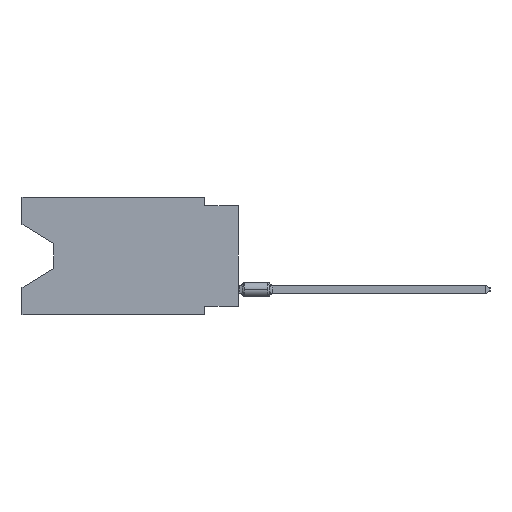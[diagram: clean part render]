
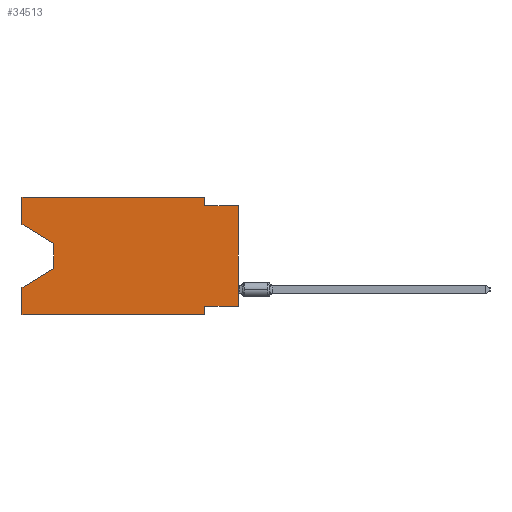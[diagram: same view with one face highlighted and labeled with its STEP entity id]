
A CAD part, left-side view. The second image highlights one B-rep face of the part: STEP entity #34513.
In plain terms, the highlighted planar face has unit normal (-1, 0, 0).
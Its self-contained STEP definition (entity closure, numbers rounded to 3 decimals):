
#129 = VECTOR ( 'NONE', #29697, 1000. ) ;
#216 = LINE ( 'NONE', #17724, #31245 ) ;
#1374 = VECTOR ( 'NONE', #54498, 1000. ) ;
#4129 = CARTESIAN_POINT ( 'NONE',  ( 0., 0., -8.255 ) ) ;
#4713 = CARTESIAN_POINT ( 'NONE',  ( 0., 16.383, -2.038 ) ) ;
#5659 = VERTEX_POINT ( 'NONE', #6612 ) ;
#6076 = EDGE_CURVE ( 'NONE', #41619, #32062, #18336, .T. ) ;
#6612 = CARTESIAN_POINT ( 'NONE',  ( 0., 13.97, -5.385 ) ) ;
#6839 = VERTEX_POINT ( 'NONE', #66470 ) ;
#8188 = LINE ( 'NONE', #26100, #9422 ) ;
#8651 = CARTESIAN_POINT ( 'NONE',  ( 0., 0., -0.635 ) ) ;
#9422 = VECTOR ( 'NONE', #55083, 1000. ) ;
#10755 = DIRECTION ( 'NONE',  ( 0., 0., -1. ) ) ;
#11193 = CARTESIAN_POINT ( 'NONE',  ( 0., 16.383, 0. ) ) ;
#12175 = ORIENTED_EDGE ( 'NONE', *, *, #22159, .F. ) ;
#12281 = VERTEX_POINT ( 'NONE', #67419 ) ;
#12905 = ORIENTED_EDGE ( 'NONE', *, *, #56607, .T. ) ;
#12911 = CARTESIAN_POINT ( 'NONE',  ( 0., 16.383, 0. ) ) ;
#13136 = EDGE_CURVE ( 'NONE', #59934, #41619, #51256, .T. ) ;
#16510 = VECTOR ( 'NONE', #16932, 1000. ) ;
#16600 = VECTOR ( 'NONE', #67827, 1000. ) ;
#16650 = EDGE_CURVE ( 'NONE', #12281, #48708, #51633, .T. ) ;
#16932 = DIRECTION ( 'NONE',  ( 0., 0., -1. ) ) ;
#17724 = CARTESIAN_POINT ( 'NONE',  ( 0., 16.383, -8.89 ) ) ;
#18336 = LINE ( 'NONE', #36245, #31512 ) ;
#19347 = ORIENTED_EDGE ( 'NONE', *, *, #30000, .F. ) ;
#19794 = CARTESIAN_POINT ( 'NONE',  ( 0., 16.383, 0. ) ) ;
#21290 = CARTESIAN_POINT ( 'NONE',  ( 0., 16.383, 0. ) ) ;
#21464 = DIRECTION ( 'NONE',  ( 1., 0., 0. ) ) ;
#22159 = EDGE_CURVE ( 'NONE', #51111, #43283, #74536, .T. ) ;
#22175 = DIRECTION ( 'NONE',  ( 0., 1., 0. ) ) ;
#22313 = AXIS2_PLACEMENT_3D ( 'NONE', #39754, #21464, #10755 ) ;
#23306 = CARTESIAN_POINT ( 'NONE',  ( 0., 0., -8.255 ) ) ;
#23835 = VERTEX_POINT ( 'NONE', #4129 ) ;
#23990 = LINE ( 'NONE', #64789, #129 ) ;
#24214 = DIRECTION ( 'NONE',  ( 0., -1., 0. ) ) ;
#25020 = ORIENTED_EDGE ( 'NONE', *, *, #69654, .F. ) ;
#25184 = DIRECTION ( 'NONE',  ( 0., 0., -1. ) ) ;
#25199 = VECTOR ( 'NONE', #74896, 1000. ) ;
#26100 = CARTESIAN_POINT ( 'NONE',  ( 0., 0., -0.635 ) ) ;
#26373 = VECTOR ( 'NONE', #22175, 1000. ) ;
#27166 = VECTOR ( 'NONE', #56360, 1000. ) ;
#29512 = ORIENTED_EDGE ( 'NONE', *, *, #6076, .F. ) ;
#29697 = DIRECTION ( 'NONE',  ( 0., 0., 1. ) ) ;
#30000 = EDGE_CURVE ( 'NONE', #23835, #51111, #51157, .T. ) ;
#31245 = VECTOR ( 'NONE', #24214, 1000. ) ;
#31512 = VECTOR ( 'NONE', #25184, 1000. ) ;
#32062 = VERTEX_POINT ( 'NONE', #60522 ) ;
#32396 = VECTOR ( 'NONE', #38109, 1000. ) ;
#33243 = ORIENTED_EDGE ( 'NONE', *, *, #13136, .F. ) ;
#34513 = ADVANCED_FACE ( 'NONE', ( #74474 ), #45465, .F. ) ;
#34594 = CARTESIAN_POINT ( 'NONE',  ( 0., 2.54, -8.89 ) ) ;
#36245 = CARTESIAN_POINT ( 'NONE',  ( 0., 2.54, 0. ) ) ;
#36279 = ORIENTED_EDGE ( 'NONE', *, *, #67643, .T. ) ;
#38109 = DIRECTION ( 'NONE',  ( 0., 0., -1. ) ) ;
#38447 = ORIENTED_EDGE ( 'NONE', *, *, #64641, .F. ) ;
#38827 = CARTESIAN_POINT ( 'NONE',  ( 0., 13.97, -5.385 ) ) ;
#39754 = CARTESIAN_POINT ( 'NONE',  ( 0., 16.383, 0. ) ) ;
#41619 = VERTEX_POINT ( 'NONE', #64195 ) ;
#43283 = VERTEX_POINT ( 'NONE', #34594 ) ;
#43777 = ORIENTED_EDGE ( 'NONE', *, *, #57644, .F. ) ;
#43829 = LINE ( 'NONE', #72840, #32396 ) ;
#44542 = LINE ( 'NONE', #38827, #27166 ) ;
#44821 = CARTESIAN_POINT ( 'NONE',  ( 0., 2.54, -8.255 ) ) ;
#45465 = PLANE ( 'NONE',  #22313 ) ;
#45922 = CARTESIAN_POINT ( 'NONE',  ( 0., 2.54, -8.89 ) ) ;
#47855 = EDGE_LOOP ( 'NONE', ( #72438, #71416, #61014, #25020, #12905, #12175, #19347, #36279, #38447, #29512, #33243, #43777 ) ) ;
#48193 = VECTOR ( 'NONE', #52026, 1000. ) ;
#48235 = CARTESIAN_POINT ( 'NONE',  ( 0., 13.97, -3.505 ) ) ;
#48708 = VERTEX_POINT ( 'NONE', #48235 ) ;
#51111 = VERTEX_POINT ( 'NONE', #44821 ) ;
#51157 = LINE ( 'NONE', #23306, #26373 ) ;
#51256 = LINE ( 'NONE', #11193, #48193 ) ;
#51411 = LINE ( 'NONE', #21290, #16600 ) ;
#51633 = LINE ( 'NONE', #4713, #25199 ) ;
#52026 = DIRECTION ( 'NONE',  ( 0., -1., 0. ) ) ;
#52636 = EDGE_CURVE ( 'NONE', #5659, #74537, #44542, .T. ) ;
#53001 = LINE ( 'NONE', #19794, #1374 ) ;
#54498 = DIRECTION ( 'NONE',  ( 0., 0., 1. ) ) ;
#55083 = DIRECTION ( 'NONE',  ( 0., -1., 0. ) ) ;
#56360 = DIRECTION ( 'NONE',  ( 0., 0.855, -0.519 ) ) ;
#56607 = EDGE_CURVE ( 'NONE', #6839, #43283, #216, .T. ) ;
#57644 = EDGE_CURVE ( 'NONE', #12281, #59934, #51411, .T. ) ;
#59934 = VERTEX_POINT ( 'NONE', #12911 ) ;
#60522 = CARTESIAN_POINT ( 'NONE',  ( 0., 2.54, -0.635 ) ) ;
#61014 = ORIENTED_EDGE ( 'NONE', *, *, #52636, .T. ) ;
#63433 = EDGE_CURVE ( 'NONE', #48708, #5659, #43829, .T. ) ;
#64195 = CARTESIAN_POINT ( 'NONE',  ( 0., 2.54, 0. ) ) ;
#64641 = EDGE_CURVE ( 'NONE', #32062, #71358, #8188, .T. ) ;
#64789 = CARTESIAN_POINT ( 'NONE',  ( 0., 0., 0. ) ) ;
#66470 = CARTESIAN_POINT ( 'NONE',  ( 0., 16.383, -8.89 ) ) ;
#67419 = CARTESIAN_POINT ( 'NONE',  ( 0., 16.383, -2.038 ) ) ;
#67643 = EDGE_CURVE ( 'NONE', #23835, #71358, #23990, .T. ) ;
#67827 = DIRECTION ( 'NONE',  ( 0., 0., 1. ) ) ;
#69654 = EDGE_CURVE ( 'NONE', #6839, #74537, #53001, .T. ) ;
#71358 = VERTEX_POINT ( 'NONE', #8651 ) ;
#71416 = ORIENTED_EDGE ( 'NONE', *, *, #63433, .T. ) ;
#72363 = CARTESIAN_POINT ( 'NONE',  ( 0., 16.383, -6.852 ) ) ;
#72438 = ORIENTED_EDGE ( 'NONE', *, *, #16650, .T. ) ;
#72840 = CARTESIAN_POINT ( 'NONE',  ( 0., 13.97, -3.505 ) ) ;
#74474 = FACE_OUTER_BOUND ( 'NONE', #47855, .T. ) ;
#74536 = LINE ( 'NONE', #45922, #16510 ) ;
#74537 = VERTEX_POINT ( 'NONE', #72363 ) ;
#74896 = DIRECTION ( 'NONE',  ( 0., -0.855, -0.519 ) ) ;
